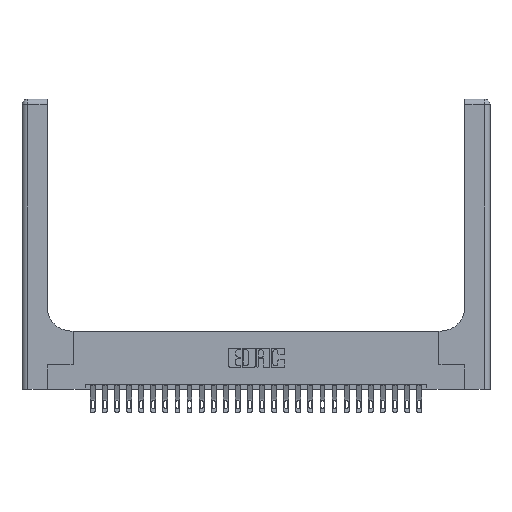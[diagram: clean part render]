
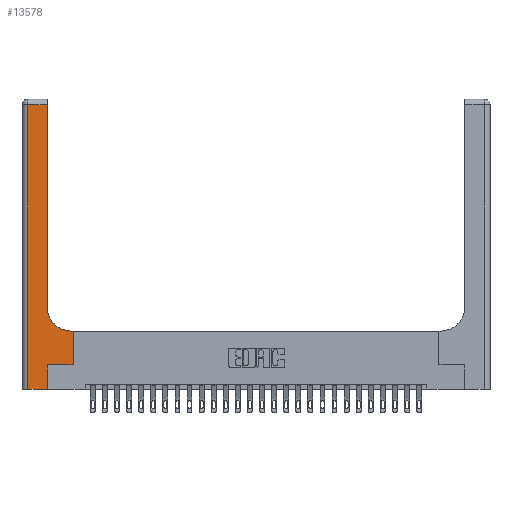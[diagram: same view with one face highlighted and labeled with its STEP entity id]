
A CAD part, top view. The second image highlights one B-rep face of the part: STEP entity #13578.
In plain terms, the highlighted planar face has unit normal (0, 0, 1).
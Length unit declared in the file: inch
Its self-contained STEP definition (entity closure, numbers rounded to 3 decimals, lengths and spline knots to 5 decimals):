
#577 = CIRCLE ( 'NONE', #17071, 0.25 ) ;
#945 = VERTEX_POINT ( 'NONE', #6000 ) ;
#1157 = CARTESIAN_POINT ( 'NONE',  ( 0.265, 0.25, 0.37 ) ) ;
#1225 = LINE ( 'NONE', #11407, #20002 ) ;
#1378 = PLANE ( 'NONE',  #23974 ) ;
#1617 = CARTESIAN_POINT ( 'NONE',  ( 0.265, 0.25, 0.37 ) ) ;
#1962 = EDGE_CURVE ( 'NONE', #6821, #14049, #18487, .T. ) ;
#2115 = CARTESIAN_POINT ( 'NONE',  ( 0., 3., 0.37 ) ) ;
#2203 = VECTOR ( 'NONE', #3611, 39.37008 ) ;
#2869 = VECTOR ( 'NONE', #2987, 39.37008 ) ;
#2987 = DIRECTION ( 'NONE',  ( 1., 0., 0. ) ) ;
#3141 = DIRECTION ( 'NONE',  ( 0., -1., 0. ) ) ;
#3357 = CARTESIAN_POINT ( 'NONE',  ( 0.265, 0., 0.37 ) ) ;
#3611 = DIRECTION ( 'NONE',  ( 0., 1., 0. ) ) ;
#4272 = CARTESIAN_POINT ( 'NONE',  ( 0.26, 2.94, 0.37 ) ) ;
#4970 = CARTESIAN_POINT ( 'NONE',  ( 0., 2.94, 0.37 ) ) ;
#5154 = EDGE_CURVE ( 'NONE', #945, #22157, #9101, .T. ) ;
#5315 = DIRECTION ( 'NONE',  ( 0., 0., -1. ) ) ;
#5686 = VERTEX_POINT ( 'NONE', #23336 ) ;
#6000 = CARTESIAN_POINT ( 'NONE',  ( 0.06, 2.94, 0.37 ) ) ;
#6463 = LINE ( 'NONE', #8575, #13609 ) ;
#6544 = CARTESIAN_POINT ( 'NONE',  ( 0.51, 0.6, 0.37 ) ) ;
#6769 = EDGE_CURVE ( 'NONE', #14049, #25872, #577, .T. ) ;
#6821 = VERTEX_POINT ( 'NONE', #13435 ) ;
#6976 = ORIENTED_EDGE ( 'NONE', *, *, #17884, .T. ) ;
#7307 = LINE ( 'NONE', #3357, #2203 ) ;
#7487 = CARTESIAN_POINT ( 'NONE',  ( 0.528, 0.25, 0.37 ) ) ;
#7948 = EDGE_LOOP ( 'NONE', ( #23315, #25678, #19547, #20029, #20741, #15311, #6976, #14278, #13657 ) ) ;
#8161 = FACE_OUTER_BOUND ( 'NONE', #7948, .T. ) ;
#8491 = VERTEX_POINT ( 'NONE', #18426 ) ;
#8575 = CARTESIAN_POINT ( 'NONE',  ( 0.26, 3., 0.37 ) ) ;
#9101 = LINE ( 'NONE', #25228, #9843 ) ;
#9778 = LINE ( 'NONE', #7487, #21622 ) ;
#9843 = VECTOR ( 'NONE', #3141, 39.37008 ) ;
#10673 = DIRECTION ( 'NONE',  ( -1., 0., 0. ) ) ;
#11407 = CARTESIAN_POINT ( 'NONE',  ( 0., 0., 0.37 ) ) ;
#11657 = DIRECTION ( 'NONE',  ( 1., 0., 0. ) ) ;
#12667 = CARTESIAN_POINT ( 'NONE',  ( 0.26, 0.6, 0.37 ) ) ;
#13183 = DIRECTION ( 'NONE',  ( 1., 0., 0. ) ) ;
#13255 = VECTOR ( 'NONE', #15042, 39.37008 ) ;
#13435 = CARTESIAN_POINT ( 'NONE',  ( 0.528, 0.6, 0.37 ) ) ;
#13578 = ADVANCED_FACE ( 'NONE', ( #8161 ), #1378, .F. ) ;
#13609 = VECTOR ( 'NONE', #14537, 39.37008 ) ;
#13653 = DIRECTION ( 'NONE',  ( -1., 0., 0. ) ) ;
#13657 = ORIENTED_EDGE ( 'NONE', *, *, #6769, .T. ) ;
#14049 = VERTEX_POINT ( 'NONE', #6544 ) ;
#14278 = ORIENTED_EDGE ( 'NONE', *, *, #1962, .T. ) ;
#14448 = VECTOR ( 'NONE', #10673, 39.37008 ) ;
#14537 = DIRECTION ( 'NONE',  ( 0., 1., 0. ) ) ;
#15042 = DIRECTION ( 'NONE',  ( -1., 0., 0. ) ) ;
#15175 = CARTESIAN_POINT ( 'NONE',  ( 0.51, 0.85, 0.37 ) ) ;
#15311 = ORIENTED_EDGE ( 'NONE', *, *, #25730, .T. ) ;
#15950 = CARTESIAN_POINT ( 'NONE',  ( 0.06, 0., 0.37 ) ) ;
#17034 = LINE ( 'NONE', #4970, #13255 ) ;
#17071 = AXIS2_PLACEMENT_3D ( 'NONE', #15175, #23220, #13183 ) ;
#17283 = VERTEX_POINT ( 'NONE', #4272 ) ;
#17542 = CARTESIAN_POINT ( 'NONE',  ( 0.26, 0.85, 0.37 ) ) ;
#17613 = EDGE_CURVE ( 'NONE', #25872, #17283, #6463, .T. ) ;
#17884 = EDGE_CURVE ( 'NONE', #5686, #6821, #9778, .T. ) ;
#18426 = CARTESIAN_POINT ( 'NONE',  ( 0.265, 0., 0.37 ) ) ;
#18487 = LINE ( 'NONE', #12667, #14448 ) ;
#18601 = EDGE_CURVE ( 'NONE', #8491, #19068, #7307, .T. ) ;
#19068 = VERTEX_POINT ( 'NONE', #1617 ) ;
#19547 = ORIENTED_EDGE ( 'NONE', *, *, #5154, .T. ) ;
#20002 = VECTOR ( 'NONE', #11657, 39.37008 ) ;
#20029 = ORIENTED_EDGE ( 'NONE', *, *, #21717, .T. ) ;
#20741 = ORIENTED_EDGE ( 'NONE', *, *, #18601, .T. ) ;
#21128 = LINE ( 'NONE', #1157, #2869 ) ;
#21622 = VECTOR ( 'NONE', #21932, 39.37008 ) ;
#21717 = EDGE_CURVE ( 'NONE', #22157, #8491, #1225, .T. ) ;
#21901 = EDGE_CURVE ( 'NONE', #17283, #945, #17034, .T. ) ;
#21932 = DIRECTION ( 'NONE',  ( 0., 1., 0. ) ) ;
#22157 = VERTEX_POINT ( 'NONE', #15950 ) ;
#23220 = DIRECTION ( 'NONE',  ( 0., 0., -1. ) ) ;
#23315 = ORIENTED_EDGE ( 'NONE', *, *, #17613, .T. ) ;
#23336 = CARTESIAN_POINT ( 'NONE',  ( 0.528, 0.25, 0.37 ) ) ;
#23974 = AXIS2_PLACEMENT_3D ( 'NONE', #2115, #5315, #13653 ) ;
#25228 = CARTESIAN_POINT ( 'NONE',  ( 0.06, 3., 0.37 ) ) ;
#25678 = ORIENTED_EDGE ( 'NONE', *, *, #21901, .T. ) ;
#25730 = EDGE_CURVE ( 'NONE', #19068, #5686, #21128, .T. ) ;
#25872 = VERTEX_POINT ( 'NONE', #17542 ) ;
